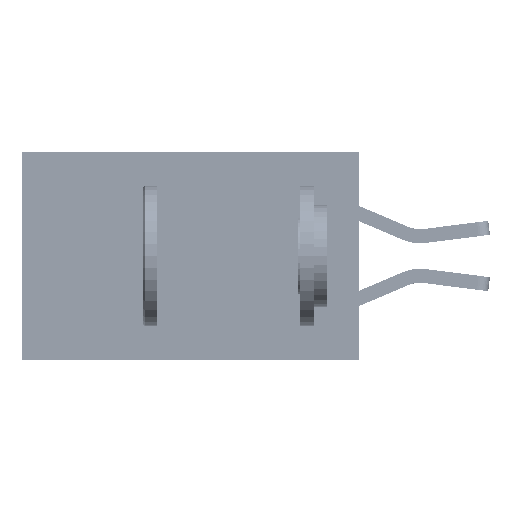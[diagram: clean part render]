
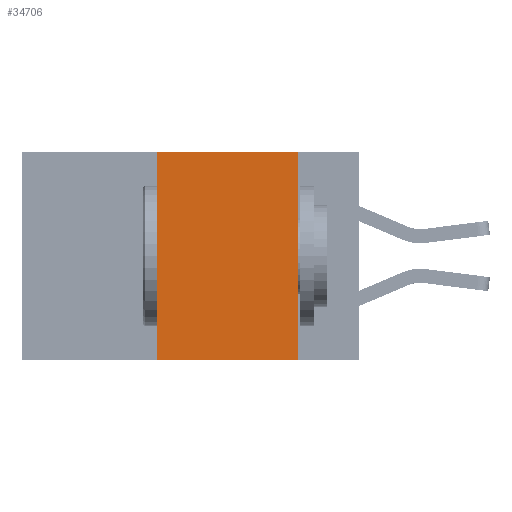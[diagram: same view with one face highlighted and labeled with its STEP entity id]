
A CAD part, left-side view. The second image highlights one B-rep face of the part: STEP entity #34706.
In plain terms, the highlighted planar face has unit normal (-1, 0, 0).
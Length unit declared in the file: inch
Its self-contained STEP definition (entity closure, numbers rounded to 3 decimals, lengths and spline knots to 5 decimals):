
#414 = EDGE_LOOP ( 'NONE', ( #15374, #20224, #17323, #28770 ) ) ;
#1131 = VECTOR ( 'NONE', #24122, 39.37008 ) ;
#4272 = CARTESIAN_POINT ( 'NONE',  ( 0., 0.36, 0. ) ) ;
#4278 = FACE_OUTER_BOUND ( 'NONE', #414, .T. ) ;
#5216 = EDGE_CURVE ( 'NONE', #26822, #25635, #28344, .T. ) ;
#5768 = AXIS2_PLACEMENT_3D ( 'NONE', #19489, #13376, #11045 ) ;
#6870 = LINE ( 'NONE', #4272, #1131 ) ;
#8024 = VECTOR ( 'NONE', #20925, 39.37008 ) ;
#8956 = EDGE_CURVE ( 'NONE', #12226, #13905, #13433, .T. ) ;
#9669 = CARTESIAN_POINT ( 'NONE',  ( 0., 0.6, -0.37 ) ) ;
#11045 = DIRECTION ( 'NONE',  ( 0., 0., -1. ) ) ;
#12226 = VERTEX_POINT ( 'NONE', #33825 ) ;
#13376 = DIRECTION ( 'NONE',  ( 1., 0., 0. ) ) ;
#13433 = LINE ( 'NONE', #36660, #29805 ) ;
#13595 = DIRECTION ( 'NONE',  ( 0., -1., 0. ) ) ;
#13905 = VERTEX_POINT ( 'NONE', #25303 ) ;
#14170 = EDGE_CURVE ( 'NONE', #13905, #25635, #32392, .T. ) ;
#15374 = ORIENTED_EDGE ( 'NONE', *, *, #14170, .F. ) ;
#16495 = CARTESIAN_POINT ( 'NONE',  ( 0., 0.11, -0.37 ) ) ;
#17323 = ORIENTED_EDGE ( 'NONE', *, *, #27721, .F. ) ;
#18200 = VECTOR ( 'NONE', #23674, 39.37008 ) ;
#19489 = CARTESIAN_POINT ( 'NONE',  ( 0., 0.6, 0. ) ) ;
#20224 = ORIENTED_EDGE ( 'NONE', *, *, #8956, .F. ) ;
#20925 = DIRECTION ( 'NONE',  ( 0., 0., -1. ) ) ;
#23276 = CARTESIAN_POINT ( 'NONE',  ( 0., 0.11, 0. ) ) ;
#23674 = DIRECTION ( 'NONE',  ( 0., -1., 0. ) ) ;
#24122 = DIRECTION ( 'NONE',  ( 0., 0., 1. ) ) ;
#25303 = CARTESIAN_POINT ( 'NONE',  ( 0., 0.11, 0. ) ) ;
#25635 = VERTEX_POINT ( 'NONE', #16495 ) ;
#26822 = VERTEX_POINT ( 'NONE', #34985 ) ;
#27721 = EDGE_CURVE ( 'NONE', #26822, #12226, #6870, .T. ) ;
#28344 = LINE ( 'NONE', #9669, #18200 ) ;
#28770 = ORIENTED_EDGE ( 'NONE', *, *, #5216, .T. ) ;
#29805 = VECTOR ( 'NONE', #13595, 39.37008 ) ;
#30337 = PLANE ( 'NONE',  #5768 ) ;
#32392 = LINE ( 'NONE', #23276, #8024 ) ;
#33825 = CARTESIAN_POINT ( 'NONE',  ( 0., 0.36, 0. ) ) ;
#34706 = ADVANCED_FACE ( 'NONE', ( #4278 ), #30337, .F. ) ;
#34985 = CARTESIAN_POINT ( 'NONE',  ( 0., 0.36, -0.37 ) ) ;
#36660 = CARTESIAN_POINT ( 'NONE',  ( 0., 0.6, 0. ) ) ;
